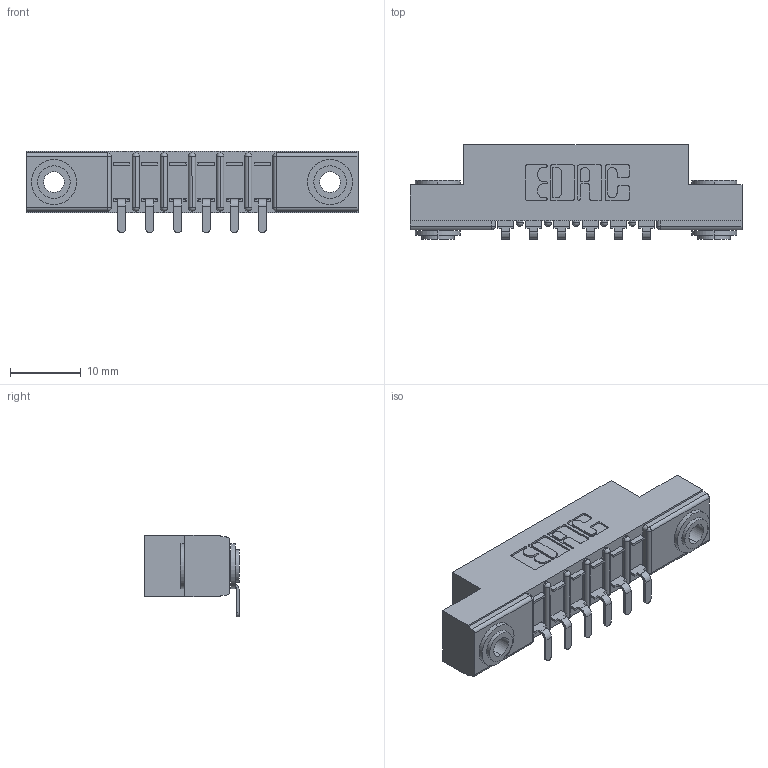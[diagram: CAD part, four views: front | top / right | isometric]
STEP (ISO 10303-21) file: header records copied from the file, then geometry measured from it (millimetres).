
FILE_DESCRIPTION (( 'STEP AP203' ), '1' );
FILE_NAME ('357-006-553-103.STEP', '2018-08-06T23:16:01', ( '' ), ( '' ), 'SwSTEP 2.0', 'SolidWorks 2016', '' );
FILE_SCHEMA (( 'CONFIG_CONTROL_DESIGN' ));
Length unit declared in the file: inch
Products named in the file (4): 307 Part_.156 Dia Mounting Holes; 307-290-002_553; 345-250-002_345-250-002-102; 357-006-553-103
Assembly tree (9 placements, depth 2):
  357-006-553-103
    307 Part_.156 Dia Mounting Holes
    307-290-002_553  x6
    345-250-002_345-250-002-102  x2
Bounding box: 46.79 x 13.36 x 11.51 mm (x, y, z)
Volume: 3081.7 mm3; surface area: 4961.2 mm2
Topology: 9 solids, 9 shells, 645 faces, 1899 edges, 1242 vertices
Faces by surface type: plane 376, cylinder 247, sphere 14, cone 8
Entity records: 11501 total; most frequent: CARTESIAN_POINT 1913, ORIENTED_EDGE 1894, DIRECTION 1891, EDGE_CURVE 947, VECTOR 699, LINE 699, VERTEX_POINT 618, AXIS2_PLACEMENT_3D 596
